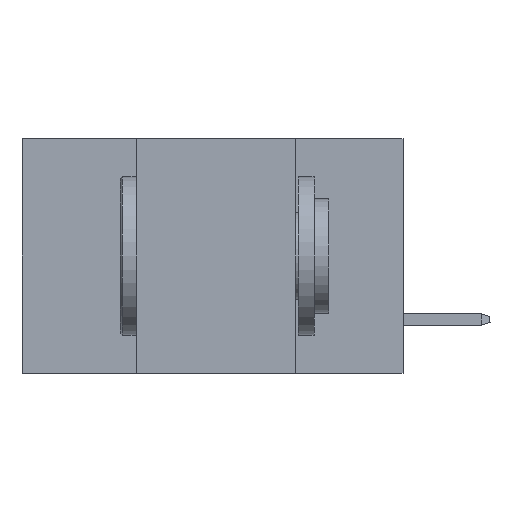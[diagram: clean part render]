
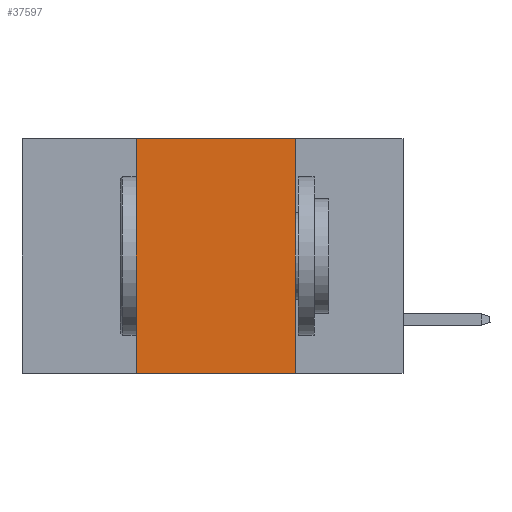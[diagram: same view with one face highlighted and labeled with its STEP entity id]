
A CAD part, left-side view. The second image highlights one B-rep face of the part: STEP entity #37597.
In plain terms, the highlighted planar face has unit normal (-1, 0, 0).
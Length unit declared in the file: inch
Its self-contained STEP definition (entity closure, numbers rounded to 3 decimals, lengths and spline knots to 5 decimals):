
#801 = VECTOR ( 'NONE', #14785, 39.37008 ) ;
#1025 = CARTESIAN_POINT ( 'NONE',  ( 0., 0.17, 0. ) ) ;
#2838 = ORIENTED_EDGE ( 'NONE', *, *, #29424, .F. ) ;
#3948 = LINE ( 'NONE', #13146, #26873 ) ;
#4247 = DIRECTION ( 'NONE',  ( 0., -1., 0. ) ) ;
#6825 = CARTESIAN_POINT ( 'NONE',  ( 0., 0.17, -0.37 ) ) ;
#7708 = EDGE_CURVE ( 'NONE', #33796, #30273, #3948, .T. ) ;
#8549 = CARTESIAN_POINT ( 'NONE',  ( 0., 0.42, 0. ) ) ;
#9426 = DIRECTION ( 'NONE',  ( 1., 0., 0. ) ) ;
#9783 = EDGE_CURVE ( 'NONE', #12971, #17900, #31047, .T. ) ;
#12241 = CARTESIAN_POINT ( 'NONE',  ( 0., 0.42, -0.37 ) ) ;
#12360 = FACE_OUTER_BOUND ( 'NONE', #29542, .T. ) ;
#12971 = VERTEX_POINT ( 'NONE', #28196 ) ;
#13146 = CARTESIAN_POINT ( 'NONE',  ( 0., 0.6, -0.37 ) ) ;
#14785 = DIRECTION ( 'NONE',  ( 0., 0., 1. ) ) ;
#15902 = DIRECTION ( 'NONE',  ( 0., -1., 0. ) ) ;
#16945 = LINE ( 'NONE', #8549, #801 ) ;
#17900 = VERTEX_POINT ( 'NONE', #1025 ) ;
#19048 = VECTOR ( 'NONE', #31150, 39.37008 ) ;
#20091 = VECTOR ( 'NONE', #4247, 39.37008 ) ;
#21121 = ORIENTED_EDGE ( 'NONE', *, *, #7708, .T. ) ;
#21390 = DIRECTION ( 'NONE',  ( 0., 0., -1. ) ) ;
#24298 = PLANE ( 'NONE',  #36956 ) ;
#24411 = CARTESIAN_POINT ( 'NONE',  ( 0., 0.6, 0. ) ) ;
#24911 = LINE ( 'NONE', #36832, #19048 ) ;
#26873 = VECTOR ( 'NONE', #15902, 39.37008 ) ;
#27069 = ORIENTED_EDGE ( 'NONE', *, *, #29099, .F. ) ;
#27395 = ORIENTED_EDGE ( 'NONE', *, *, #9783, .F. ) ;
#28196 = CARTESIAN_POINT ( 'NONE',  ( 0., 0.42, 0. ) ) ;
#29099 = EDGE_CURVE ( 'NONE', #33796, #12971, #16945, .T. ) ;
#29424 = EDGE_CURVE ( 'NONE', #17900, #30273, #24911, .T. ) ;
#29542 = EDGE_LOOP ( 'NONE', ( #2838, #27395, #27069, #21121 ) ) ;
#30273 = VERTEX_POINT ( 'NONE', #6825 ) ;
#31047 = LINE ( 'NONE', #24411, #20091 ) ;
#31150 = DIRECTION ( 'NONE',  ( 0., 0., -1. ) ) ;
#33796 = VERTEX_POINT ( 'NONE', #12241 ) ;
#36210 = CARTESIAN_POINT ( 'NONE',  ( 0., 0.6, 0. ) ) ;
#36832 = CARTESIAN_POINT ( 'NONE',  ( 0., 0.17, 0. ) ) ;
#36956 = AXIS2_PLACEMENT_3D ( 'NONE', #36210, #9426, #21390 ) ;
#37597 = ADVANCED_FACE ( 'NONE', ( #12360 ), #24298, .F. ) ;
